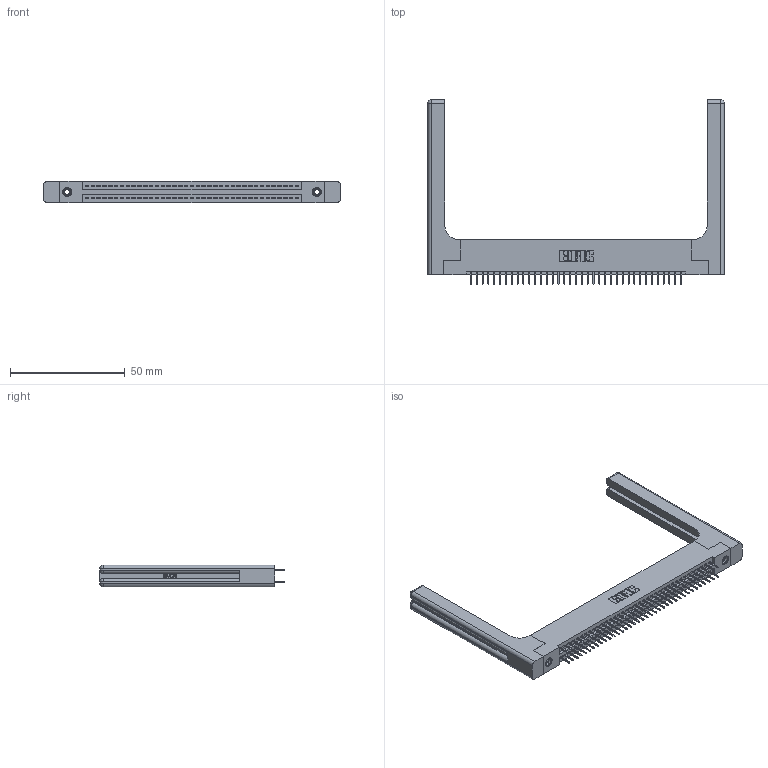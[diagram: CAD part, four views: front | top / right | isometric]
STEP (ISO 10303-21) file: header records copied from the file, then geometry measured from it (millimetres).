
FILE_DESCRIPTION (( 'STEP AP203' ), '1' );
FILE_NAME ('395-074-524-258.STEP', '2019-10-24T14:04:27', ( '' ), ( '' ), 'SwSTEP 2.0', 'SolidWorks 2016', '' );
FILE_SCHEMA (( 'CONFIG_CONTROL_DESIGN' ));
Length unit declared in the file: inch
Products named in the file (5): 345-292-001_345-293-124; 345-250-001_345-250-001-102; 345-220-058_345-220-058; 395-074-524-258; 345 Part_Flush Mounting Lugs - 0.156 Dia-TH
Assembly tree (79 placements, depth 2):
  395-074-524-258
    345 Part_Flush Mounting Lugs - 0.156 Dia-TH
    345-292-001_345-293-124  x74
    345-250-001_345-250-001-102  x2
    345-220-058_345-220-058  x2
Bounding box: 129.01 x 80.31 x 9.4 mm (x, y, z)
Volume: 20848.5 mm3; surface area: 22956.4 mm2
Topology: 79 solids, 79 shells, 4378 faces, 12329 edges, 7902 vertices
Faces by surface type: plane 3114, cylinder 1204, bspline 36, cone 12, sphere 8, torus 4
Entity records: 34960 total; most frequent: CARTESIAN_POINT 6857, ORIENTED_EDGE 5588, DIRECTION 4986, EDGE_CURVE 2794, VECTOR 2426, LINE 2426, VERTEX_POINT 1850, AXIS2_PLACEMENT_3D 1280
